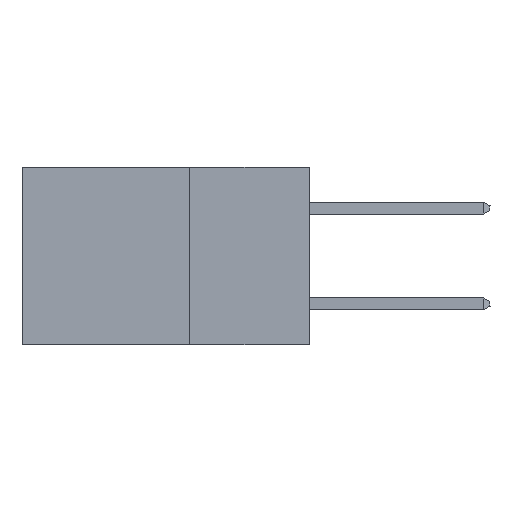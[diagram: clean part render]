
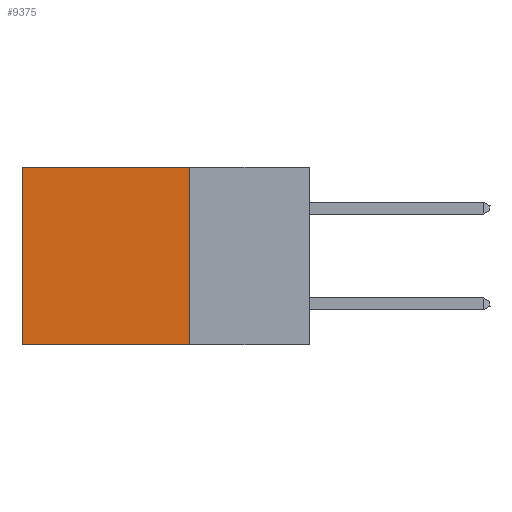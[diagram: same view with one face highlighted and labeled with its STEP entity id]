
A CAD part, left-side view. The second image highlights one B-rep face of the part: STEP entity #9375.
In plain terms, the highlighted planar face has unit normal (-1, 0, 0).
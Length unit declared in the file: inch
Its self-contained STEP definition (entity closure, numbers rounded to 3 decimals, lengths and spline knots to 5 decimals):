
#199 = VECTOR ( 'NONE', #17936, 39.37008 ) ;
#490 = PLANE ( 'NONE',  #8860 ) ;
#669 = CARTESIAN_POINT ( 'NONE',  ( 0.2875, 0.25, -0.37 ) ) ;
#1021 = EDGE_CURVE ( 'NONE', #4635, #14269, #1684, .T. ) ;
#1684 = LINE ( 'NONE', #669, #26184 ) ;
#1869 = VERTEX_POINT ( 'NONE', #18971 ) ;
#3653 = CARTESIAN_POINT ( 'NONE',  ( 0.2875, 0.25, 0. ) ) ;
#4632 = DIRECTION ( 'NONE',  ( 0., 0., -1. ) ) ;
#4635 = VERTEX_POINT ( 'NONE', #5139 ) ;
#4885 = VECTOR ( 'NONE', #21377, 39.37008 ) ;
#5139 = CARTESIAN_POINT ( 'NONE',  ( 0.2875, 0.25, -0.37 ) ) ;
#6952 = VERTEX_POINT ( 'NONE', #16463 ) ;
#8860 = AXIS2_PLACEMENT_3D ( 'NONE', #14832, #16877, #4632 ) ;
#9375 = ADVANCED_FACE ( 'NONE', ( #24953 ), #490, .F. ) ;
#9546 = EDGE_CURVE ( 'NONE', #6952, #14269, #17035, .T. ) ;
#12348 = EDGE_CURVE ( 'NONE', #1869, #4635, #20185, .T. ) ;
#13245 = ORIENTED_EDGE ( 'NONE', *, *, #1021, .F. ) ;
#14157 = VECTOR ( 'NONE', #15719, 39.37008 ) ;
#14269 = VERTEX_POINT ( 'NONE', #16265 ) ;
#14832 = CARTESIAN_POINT ( 'NONE',  ( 0.2875, 0.25, 0. ) ) ;
#15719 = DIRECTION ( 'NONE',  ( 0., 0., -1. ) ) ;
#16006 = ORIENTED_EDGE ( 'NONE', *, *, #12348, .F. ) ;
#16265 = CARTESIAN_POINT ( 'NONE',  ( 0.2875, 0.6, -0.37 ) ) ;
#16463 = CARTESIAN_POINT ( 'NONE',  ( 0.2875, 0.6, 0. ) ) ;
#16877 = DIRECTION ( 'NONE',  ( 1., 0., 0. ) ) ;
#17035 = LINE ( 'NONE', #19358, #4885 ) ;
#17536 = EDGE_CURVE ( 'NONE', #1869, #6952, #21278, .T. ) ;
#17559 = ORIENTED_EDGE ( 'NONE', *, *, #9546, .T. ) ;
#17936 = DIRECTION ( 'NONE',  ( 0., 1., 0. ) ) ;
#18971 = CARTESIAN_POINT ( 'NONE',  ( 0.2875, 0.25, 0. ) ) ;
#19358 = CARTESIAN_POINT ( 'NONE',  ( 0.2875, 0.6, 0. ) ) ;
#20185 = LINE ( 'NONE', #21738, #14157 ) ;
#20965 = DIRECTION ( 'NONE',  ( 0., 1., 0. ) ) ;
#21278 = LINE ( 'NONE', #3653, #199 ) ;
#21377 = DIRECTION ( 'NONE',  ( 0., 0., -1. ) ) ;
#21717 = EDGE_LOOP ( 'NONE', ( #17559, #13245, #16006, #23709 ) ) ;
#21738 = CARTESIAN_POINT ( 'NONE',  ( 0.2875, 0.25, 0. ) ) ;
#23709 = ORIENTED_EDGE ( 'NONE', *, *, #17536, .T. ) ;
#24953 = FACE_OUTER_BOUND ( 'NONE', #21717, .T. ) ;
#26184 = VECTOR ( 'NONE', #20965, 39.37008 ) ;
